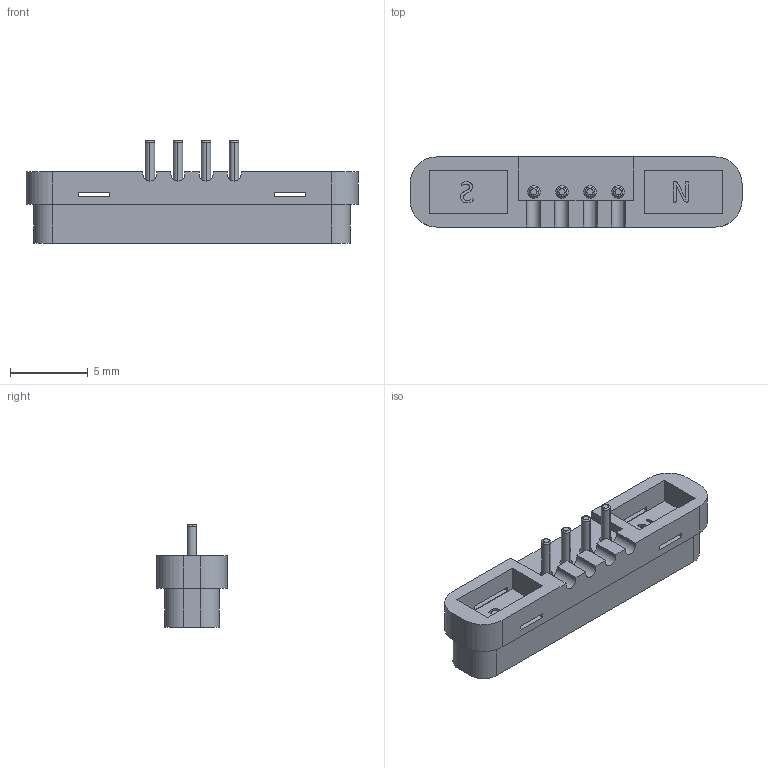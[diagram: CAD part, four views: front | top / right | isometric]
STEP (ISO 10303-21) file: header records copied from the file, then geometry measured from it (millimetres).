
FILE_DESCRIPTION (( 'STEP AP214' ), '1' );
FILE_NAME ('686C0422250110E.STEP', '2023-05-29T17:07:04', ( '' ), ( '' ), 'SwSTEP 2.0', 'SolidWorks 2020', '' );
FILE_SCHEMA (( 'AUTOMOTIVE_DESIGN' ));
Length unit declared in the file: millimetre
Products named in the file (1): 686C0422250110E
Bounding box: 21.3 x 4.5 x 6.6 mm (x, y, z)
Volume: 283.7 mm3; surface area: 600 mm2
Topology: 1 solids, 1 shells, 237 faces, 639 edges, 422 vertices
Faces by surface type: plane 130, bspline 48, cylinder 40, cone 11, torus 8
Entity records: 10746 total; most frequent: CARTESIAN_POINT 3852, ORIENTED_EDGE 1278, DIRECTION 1045, EDGE_CURVE 639, VERTEX_POINT 422, VECTOR 421, LINE 421, AXIS2_PLACEMENT_3D 312
